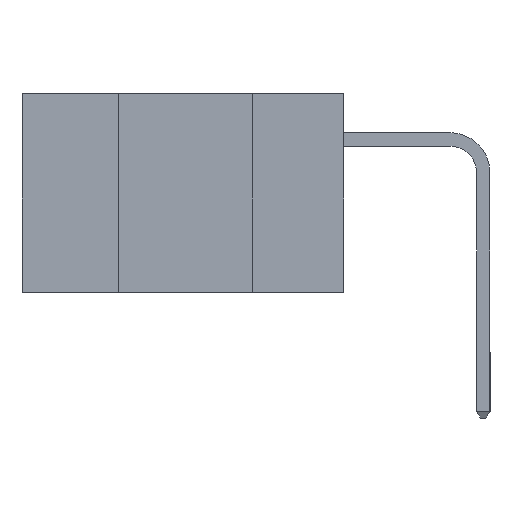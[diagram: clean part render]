
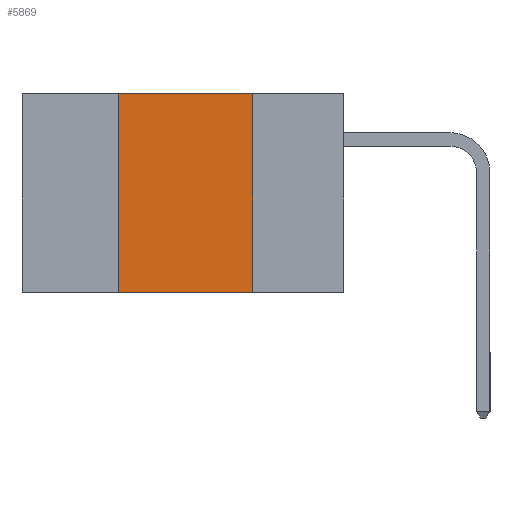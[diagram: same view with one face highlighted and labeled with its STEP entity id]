
A CAD part, left-side view. The second image highlights one B-rep face of the part: STEP entity #5869.
In plain terms, the highlighted planar face has unit normal (-1, 0, 0).
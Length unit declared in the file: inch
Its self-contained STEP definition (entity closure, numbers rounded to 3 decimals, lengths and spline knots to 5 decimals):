
#64 = CARTESIAN_POINT ( 'NONE',  ( 0., 0.17, -0.37 ) ) ;
#731 = EDGE_CURVE ( 'NONE', #2443, #4888, #11258, .T. ) ;
#1154 = ORIENTED_EDGE ( 'NONE', *, *, #6406, .F. ) ;
#1578 = DIRECTION ( 'NONE',  ( 0., 0., 1. ) ) ;
#1794 = LINE ( 'NONE', #11748, #8267 ) ;
#1853 = EDGE_CURVE ( 'NONE', #6813, #4888, #7854, .T. ) ;
#2118 = CARTESIAN_POINT ( 'NONE',  ( 0., 0.17, 0. ) ) ;
#2443 = VERTEX_POINT ( 'NONE', #2118 ) ;
#3182 = VECTOR ( 'NONE', #1578, 39.37008 ) ;
#3846 = DIRECTION ( 'NONE',  ( 0., 0., -1. ) ) ;
#3878 = VECTOR ( 'NONE', #7912, 39.37008 ) ;
#4144 = PLANE ( 'NONE',  #8954 ) ;
#4888 = VERTEX_POINT ( 'NONE', #64 ) ;
#5257 = CARTESIAN_POINT ( 'NONE',  ( 0., 0.6, -0.37 ) ) ;
#5722 = ORIENTED_EDGE ( 'NONE', *, *, #9489, .F. ) ;
#5862 = ORIENTED_EDGE ( 'NONE', *, *, #1853, .T. ) ;
#5869 = ADVANCED_FACE ( 'NONE', ( #11317 ), #4144, .F. ) ;
#6056 = ORIENTED_EDGE ( 'NONE', *, *, #731, .F. ) ;
#6406 = EDGE_CURVE ( 'NONE', #6813, #11864, #11051, .T. ) ;
#6481 = CARTESIAN_POINT ( 'NONE',  ( 0., 0.42, -0.37 ) ) ;
#6565 = CARTESIAN_POINT ( 'NONE',  ( 0., 0.17, -0.37 ) ) ;
#6813 = VERTEX_POINT ( 'NONE', #10501 ) ;
#6925 = DIRECTION ( 'NONE',  ( 0., 0., -1. ) ) ;
#7854 = LINE ( 'NONE', #5257, #3878 ) ;
#7912 = DIRECTION ( 'NONE',  ( 0., -1., 0. ) ) ;
#8124 = CARTESIAN_POINT ( 'NONE',  ( 0., 0.42, 0. ) ) ;
#8267 = VECTOR ( 'NONE', #11804, 39.37008 ) ;
#8677 = CARTESIAN_POINT ( 'NONE',  ( 0., 0.6, 0. ) ) ;
#8954 = AXIS2_PLACEMENT_3D ( 'NONE', #8677, #10414, #6925 ) ;
#9489 = EDGE_CURVE ( 'NONE', #11864, #2443, #1794, .T. ) ;
#9827 = VECTOR ( 'NONE', #3846, 39.37008 ) ;
#10414 = DIRECTION ( 'NONE',  ( 1., 0., 0. ) ) ;
#10501 = CARTESIAN_POINT ( 'NONE',  ( 0., 0.42, -0.37 ) ) ;
#11051 = LINE ( 'NONE', #6481, #3182 ) ;
#11258 = LINE ( 'NONE', #6565, #9827 ) ;
#11317 = FACE_OUTER_BOUND ( 'NONE', #11839, .T. ) ;
#11748 = CARTESIAN_POINT ( 'NONE',  ( 0., 0.6, 0. ) ) ;
#11804 = DIRECTION ( 'NONE',  ( 0., -1., 0. ) ) ;
#11839 = EDGE_LOOP ( 'NONE', ( #6056, #5722, #1154, #5862 ) ) ;
#11864 = VERTEX_POINT ( 'NONE', #8124 ) ;
